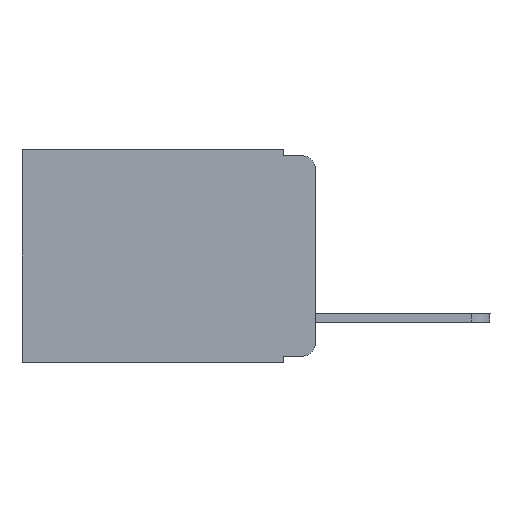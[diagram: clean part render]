
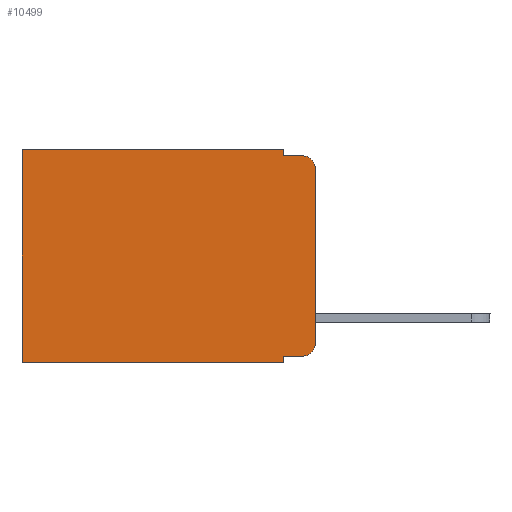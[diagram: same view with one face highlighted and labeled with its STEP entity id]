
A CAD part, left-side view. The second image highlights one B-rep face of the part: STEP entity #10499.
In plain terms, the highlighted planar face has unit normal (-1, 0, 0).
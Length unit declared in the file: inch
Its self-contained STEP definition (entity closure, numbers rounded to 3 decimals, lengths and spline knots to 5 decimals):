
#240 = EDGE_CURVE ( 'NONE', #3098, #18915, #16642, .T. ) ;
#432 = LINE ( 'NONE', #6722, #20998 ) ;
#559 = VECTOR ( 'NONE', #14294, 39.37008 ) ;
#817 = CARTESIAN_POINT ( 'NONE',  ( 0.298, 0.02, -0.01 ) ) ;
#1040 = DIRECTION ( 'NONE',  ( 0., 0., -1. ) ) ;
#1238 = DIRECTION ( 'NONE',  ( -1., 0., 0. ) ) ;
#1360 = LINE ( 'NONE', #6189, #559 ) ;
#1513 = ORIENTED_EDGE ( 'NONE', *, *, #16517, .F. ) ;
#1517 = EDGE_CURVE ( 'NONE', #11753, #5472, #6163, .T. ) ;
#1520 = EDGE_CURVE ( 'NONE', #2731, #17585, #1360, .T. ) ;
#2383 = VERTEX_POINT ( 'NONE', #817 ) ;
#2493 = PLANE ( 'NONE',  #14395 ) ;
#2731 = VERTEX_POINT ( 'NONE', #15517 ) ;
#2897 = VECTOR ( 'NONE', #17997, 39.37008 ) ;
#2946 = CARTESIAN_POINT ( 'NONE',  ( 0.298, 0.02, -0.313 ) ) ;
#3037 = ORIENTED_EDGE ( 'NONE', *, *, #1520, .T. ) ;
#3098 = VERTEX_POINT ( 'NONE', #19174 ) ;
#3160 = DIRECTION ( 'NONE',  ( 0., 0., -1. ) ) ;
#3628 = CARTESIAN_POINT ( 'NONE',  ( 0.298, 0.051, -0.343 ) ) ;
#3830 = DIRECTION ( 'NONE',  ( 1., 0., 0. ) ) ;
#3859 = ORIENTED_EDGE ( 'NONE', *, *, #240, .F. ) ;
#3982 = CARTESIAN_POINT ( 'NONE',  ( 0.298, 0., -0.313 ) ) ;
#4587 = LINE ( 'NONE', #9338, #6832 ) ;
#4699 = VERTEX_POINT ( 'NONE', #11261 ) ;
#4716 = VECTOR ( 'NONE', #1040, 39.37008 ) ;
#5230 = CARTESIAN_POINT ( 'NONE',  ( 0.298, 0.02, -0.333 ) ) ;
#5460 = CARTESIAN_POINT ( 'NONE',  ( 0.298, 0., 0. ) ) ;
#5470 = ORIENTED_EDGE ( 'NONE', *, *, #1517, .T. ) ;
#5472 = VERTEX_POINT ( 'NONE', #3982 ) ;
#5996 = CARTESIAN_POINT ( 'NONE',  ( 0.298, 0.051, -0.333 ) ) ;
#6130 = CARTESIAN_POINT ( 'NONE',  ( 0.298, 0.02, -0.03 ) ) ;
#6163 = CIRCLE ( 'NONE', #11392, 0.02 ) ;
#6189 = CARTESIAN_POINT ( 'NONE',  ( 0.298, 0., 0. ) ) ;
#6309 = ORIENTED_EDGE ( 'NONE', *, *, #14514, .T. ) ;
#6393 = ORIENTED_EDGE ( 'NONE', *, *, #18313, .F. ) ;
#6660 = DIRECTION ( 'NONE',  ( 0., 0., -1. ) ) ;
#6722 = CARTESIAN_POINT ( 'NONE',  ( 0.298, 0.473, 0. ) ) ;
#6832 = VECTOR ( 'NONE', #14013, 39.37008 ) ;
#7489 = ORIENTED_EDGE ( 'NONE', *, *, #20289, .T. ) ;
#8427 = CARTESIAN_POINT ( 'NONE',  ( 0.298, 0.051, 0. ) ) ;
#8775 = VECTOR ( 'NONE', #19001, 39.37008 ) ;
#8816 = CARTESIAN_POINT ( 'NONE',  ( 0.298, 0.473, 0. ) ) ;
#9338 = CARTESIAN_POINT ( 'NONE',  ( 0.298, 0., -0.343 ) ) ;
#10499 = ADVANCED_FACE ( 'NONE', ( #13070 ), #2493, .F. ) ;
#10530 = LINE ( 'NONE', #8427, #11516 ) ;
#11261 = CARTESIAN_POINT ( 'NONE',  ( 0.298, 0.051, -0.01 ) ) ;
#11392 = AXIS2_PLACEMENT_3D ( 'NONE', #2946, #1238, #3160 ) ;
#11410 = LINE ( 'NONE', #12393, #4716 ) ;
#11516 = VECTOR ( 'NONE', #6660, 39.37008 ) ;
#11753 = VERTEX_POINT ( 'NONE', #5230 ) ;
#11763 = CARTESIAN_POINT ( 'NONE',  ( 0.298, 0., -0.03 ) ) ;
#12073 = EDGE_CURVE ( 'NONE', #3098, #11753, #20880, .T. ) ;
#12393 = CARTESIAN_POINT ( 'NONE',  ( 0.298, 0., 0. ) ) ;
#12626 = ORIENTED_EDGE ( 'NONE', *, *, #15886, .F. ) ;
#13070 = FACE_OUTER_BOUND ( 'NONE', #14636, .T. ) ;
#13488 = EDGE_CURVE ( 'NONE', #18915, #15332, #4587, .T. ) ;
#14013 = DIRECTION ( 'NONE',  ( 0., 1., 0. ) ) ;
#14294 = DIRECTION ( 'NONE',  ( 0., 1., 0. ) ) ;
#14395 = AXIS2_PLACEMENT_3D ( 'NONE', #5460, #3830, #20002 ) ;
#14514 = EDGE_CURVE ( 'NONE', #18808, #2383, #16928, .T. ) ;
#14636 = EDGE_LOOP ( 'NONE', ( #6393, #6309, #1513, #12626, #3037, #7489, #15551, #3859, #15899, #5470 ) ) ;
#15332 = VERTEX_POINT ( 'NONE', #16041 ) ;
#15517 = CARTESIAN_POINT ( 'NONE',  ( 0.298, 0.051, 0. ) ) ;
#15537 = CARTESIAN_POINT ( 'NONE',  ( 0.298, 0.051, 0. ) ) ;
#15551 = ORIENTED_EDGE ( 'NONE', *, *, #13488, .F. ) ;
#15864 = DIRECTION ( 'NONE',  ( 0., -1., 0. ) ) ;
#15875 = DIRECTION ( 'NONE',  ( -1., 0., 0. ) ) ;
#15886 = EDGE_CURVE ( 'NONE', #2731, #4699, #10530, .T. ) ;
#15899 = ORIENTED_EDGE ( 'NONE', *, *, #12073, .T. ) ;
#16041 = CARTESIAN_POINT ( 'NONE',  ( 0.298, 0.473, -0.343 ) ) ;
#16401 = CARTESIAN_POINT ( 'NONE',  ( 0.298, 0.051, -0.01 ) ) ;
#16517 = EDGE_CURVE ( 'NONE', #4699, #2383, #18087, .T. ) ;
#16642 = LINE ( 'NONE', #15537, #8775 ) ;
#16729 = AXIS2_PLACEMENT_3D ( 'NONE', #6130, #15875, #17467 ) ;
#16928 = CIRCLE ( 'NONE', #16729, 0.02 ) ;
#17467 = DIRECTION ( 'NONE',  ( 0., 0., -1. ) ) ;
#17585 = VERTEX_POINT ( 'NONE', #8816 ) ;
#17997 = DIRECTION ( 'NONE',  ( 0., -1., 0. ) ) ;
#18087 = LINE ( 'NONE', #16401, #2897 ) ;
#18313 = EDGE_CURVE ( 'NONE', #18808, #5472, #11410, .T. ) ;
#18808 = VERTEX_POINT ( 'NONE', #11763 ) ;
#18915 = VERTEX_POINT ( 'NONE', #3628 ) ;
#19001 = DIRECTION ( 'NONE',  ( 0., 0., -1. ) ) ;
#19174 = CARTESIAN_POINT ( 'NONE',  ( 0.298, 0.051, -0.333 ) ) ;
#19721 = DIRECTION ( 'NONE',  ( 0., 0., -1. ) ) ;
#20002 = DIRECTION ( 'NONE',  ( 0., 0., -1. ) ) ;
#20139 = VECTOR ( 'NONE', #15864, 39.37008 ) ;
#20289 = EDGE_CURVE ( 'NONE', #17585, #15332, #432, .T. ) ;
#20880 = LINE ( 'NONE', #5996, #20139 ) ;
#20998 = VECTOR ( 'NONE', #19721, 39.37008 ) ;
